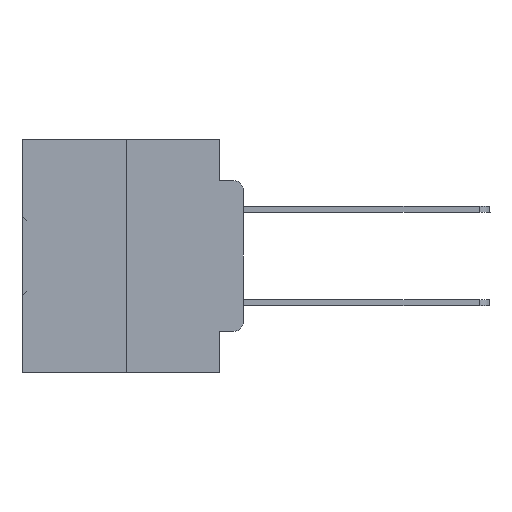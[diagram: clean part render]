
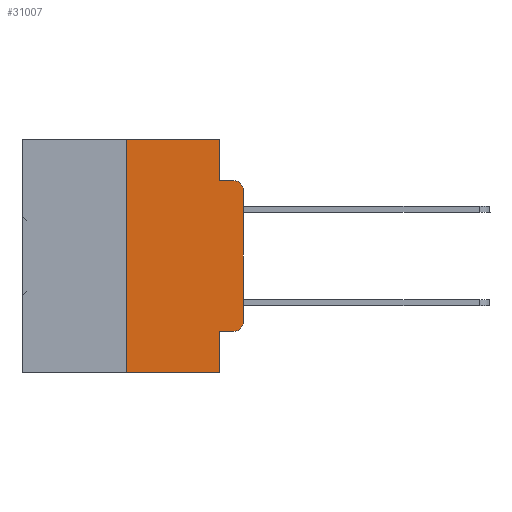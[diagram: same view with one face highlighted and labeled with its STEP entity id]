
A CAD part, left-side view. The second image highlights one B-rep face of the part: STEP entity #31007.
In plain terms, the highlighted planar face has unit normal (-1, 0, 0).
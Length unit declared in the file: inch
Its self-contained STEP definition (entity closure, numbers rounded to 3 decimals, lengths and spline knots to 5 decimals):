
#98 = CARTESIAN_POINT ( 'NONE',  ( 0., 0.473, -0.5 ) ) ;
#1032 = CARTESIAN_POINT ( 'NONE',  ( 0., 0.051, -0.5 ) ) ;
#1757 = EDGE_LOOP ( 'NONE', ( #6483, #30532, #11226, #21623, #28523, #35067, #13633, #14797, #33017, #24942 ) ) ;
#1871 = CARTESIAN_POINT ( 'NONE',  ( 0., 0.051, -0.0885 ) ) ;
#2220 = DIRECTION ( 'NONE',  ( 0., 0., -1. ) ) ;
#3205 = DIRECTION ( 'NONE',  ( 0., -1., 0. ) ) ;
#3514 = CARTESIAN_POINT ( 'NONE',  ( 0., 0.051, 0. ) ) ;
#3986 = CARTESIAN_POINT ( 'NONE',  ( 0., 0.02, -0.1085 ) ) ;
#4197 = VECTOR ( 'NONE', #20600, 39.37008 ) ;
#4476 = EDGE_CURVE ( 'NONE', #23168, #31035, #20911, .T. ) ;
#4956 = LINE ( 'NONE', #15078, #26193 ) ;
#5874 = EDGE_CURVE ( 'NONE', #37020, #7600, #14999, .T. ) ;
#6229 = DIRECTION ( 'NONE',  ( 0., -1., 0. ) ) ;
#6483 = ORIENTED_EDGE ( 'NONE', *, *, #4476, .T. ) ;
#6563 = CARTESIAN_POINT ( 'NONE',  ( 0., 0.473, 0. ) ) ;
#7600 = VERTEX_POINT ( 'NONE', #1032 ) ;
#8075 = VECTOR ( 'NONE', #35245, 39.37008 ) ;
#8565 = CARTESIAN_POINT ( 'NONE',  ( 0., 0.051, 0. ) ) ;
#9531 = CARTESIAN_POINT ( 'NONE',  ( 0., 0.25, -0.5 ) ) ;
#10340 = VECTOR ( 'NONE', #3205, 39.37008 ) ;
#11226 = ORIENTED_EDGE ( 'NONE', *, *, #23329, .F. ) ;
#11443 = CARTESIAN_POINT ( 'NONE',  ( 0., 0., -0.3915 ) ) ;
#11628 = CARTESIAN_POINT ( 'NONE',  ( 0., 0.473, 0. ) ) ;
#11933 = CIRCLE ( 'NONE', #19474, 0.02 ) ;
#12114 = VERTEX_POINT ( 'NONE', #34122 ) ;
#12653 = VERTEX_POINT ( 'NONE', #32882 ) ;
#13633 = ORIENTED_EDGE ( 'NONE', *, *, #5874, .T. ) ;
#13936 = LINE ( 'NONE', #15001, #8075 ) ;
#14797 = ORIENTED_EDGE ( 'NONE', *, *, #17668, .F. ) ;
#14999 = LINE ( 'NONE', #98, #29431 ) ;
#15001 = CARTESIAN_POINT ( 'NONE',  ( 0., 0.25, 0. ) ) ;
#15078 = CARTESIAN_POINT ( 'NONE',  ( 0., 0.051, -0.0885 ) ) ;
#15284 = PLANE ( 'NONE',  #18612 ) ;
#15452 = LINE ( 'NONE', #8565, #16367 ) ;
#15749 = DIRECTION ( 'NONE',  ( 0., 0., -1. ) ) ;
#16367 = VECTOR ( 'NONE', #36884, 39.37008 ) ;
#16487 = EDGE_CURVE ( 'NONE', #31035, #12114, #25071, .T. ) ;
#16771 = VERTEX_POINT ( 'NONE', #3514 ) ;
#17106 = EDGE_CURVE ( 'NONE', #33822, #16771, #24101, .T. ) ;
#17474 = CARTESIAN_POINT ( 'NONE',  ( 0., 0.051, -0.4115 ) ) ;
#17668 = EDGE_CURVE ( 'NONE', #12653, #7600, #15452, .T. ) ;
#18612 = AXIS2_PLACEMENT_3D ( 'NONE', #6563, #35014, #29514 ) ;
#19340 = DIRECTION ( 'NONE',  ( 0., 0., -1. ) ) ;
#19474 = AXIS2_PLACEMENT_3D ( 'NONE', #25005, #36799, #19340 ) ;
#19604 = VECTOR ( 'NONE', #21815, 39.37008 ) ;
#19637 = EDGE_CURVE ( 'NONE', #16771, #32309, #36359, .T. ) ;
#20600 = DIRECTION ( 'NONE',  ( 0., -1., 0. ) ) ;
#20911 = LINE ( 'NONE', #36246, #19604 ) ;
#21187 = CARTESIAN_POINT ( 'NONE',  ( 0., 0.25, 0. ) ) ;
#21623 = ORIENTED_EDGE ( 'NONE', *, *, #19637, .F. ) ;
#21815 = DIRECTION ( 'NONE',  ( 0., 0., 1. ) ) ;
#22430 = CARTESIAN_POINT ( 'NONE',  ( 0., 0.051, 0. ) ) ;
#23168 = VERTEX_POINT ( 'NONE', #11443 ) ;
#23329 = EDGE_CURVE ( 'NONE', #32309, #12114, #4956, .T. ) ;
#23826 = CARTESIAN_POINT ( 'NONE',  ( 0., 0.02, -0.4115 ) ) ;
#24101 = LINE ( 'NONE', #11628, #4197 ) ;
#24942 = ORIENTED_EDGE ( 'NONE', *, *, #25588, .T. ) ;
#25005 = CARTESIAN_POINT ( 'NONE',  ( 0., 0.02, -0.3915 ) ) ;
#25071 = CIRCLE ( 'NONE', #29871, 0.02 ) ;
#25588 = EDGE_CURVE ( 'NONE', #33699, #23168, #11933, .T. ) ;
#26193 = VECTOR ( 'NONE', #6229, 39.37008 ) ;
#27205 = DIRECTION ( 'NONE',  ( -1., 0., 0. ) ) ;
#27380 = FACE_OUTER_BOUND ( 'NONE', #1757, .T. ) ;
#28407 = LINE ( 'NONE', #17474, #10340 ) ;
#28523 = ORIENTED_EDGE ( 'NONE', *, *, #17106, .F. ) ;
#29431 = VECTOR ( 'NONE', #32081, 39.37008 ) ;
#29514 = DIRECTION ( 'NONE',  ( 0., 0., -1. ) ) ;
#29871 = AXIS2_PLACEMENT_3D ( 'NONE', #3986, #27205, #15749 ) ;
#30532 = ORIENTED_EDGE ( 'NONE', *, *, #16487, .T. ) ;
#30928 = VECTOR ( 'NONE', #2220, 39.37008 ) ;
#31007 = ADVANCED_FACE ( 'NONE', ( #27380 ), #15284, .F. ) ;
#31035 = VERTEX_POINT ( 'NONE', #32258 ) ;
#32081 = DIRECTION ( 'NONE',  ( 0., -1., 0. ) ) ;
#32258 = CARTESIAN_POINT ( 'NONE',  ( 0., 0., -0.1085 ) ) ;
#32309 = VERTEX_POINT ( 'NONE', #1871 ) ;
#32882 = CARTESIAN_POINT ( 'NONE',  ( 0., 0.051, -0.4115 ) ) ;
#33017 = ORIENTED_EDGE ( 'NONE', *, *, #35079, .T. ) ;
#33699 = VERTEX_POINT ( 'NONE', #23826 ) ;
#33822 = VERTEX_POINT ( 'NONE', #21187 ) ;
#34122 = CARTESIAN_POINT ( 'NONE',  ( 0., 0.02, -0.0885 ) ) ;
#35014 = DIRECTION ( 'NONE',  ( 1., 0., 0. ) ) ;
#35067 = ORIENTED_EDGE ( 'NONE', *, *, #36460, .F. ) ;
#35079 = EDGE_CURVE ( 'NONE', #12653, #33699, #28407, .T. ) ;
#35245 = DIRECTION ( 'NONE',  ( 0., 0., 1. ) ) ;
#36246 = CARTESIAN_POINT ( 'NONE',  ( 0., 0., 0. ) ) ;
#36359 = LINE ( 'NONE', #22430, #30928 ) ;
#36460 = EDGE_CURVE ( 'NONE', #37020, #33822, #13936, .T. ) ;
#36799 = DIRECTION ( 'NONE',  ( -1., 0., 0. ) ) ;
#36884 = DIRECTION ( 'NONE',  ( 0., 0., -1. ) ) ;
#37020 = VERTEX_POINT ( 'NONE', #9531 ) ;
